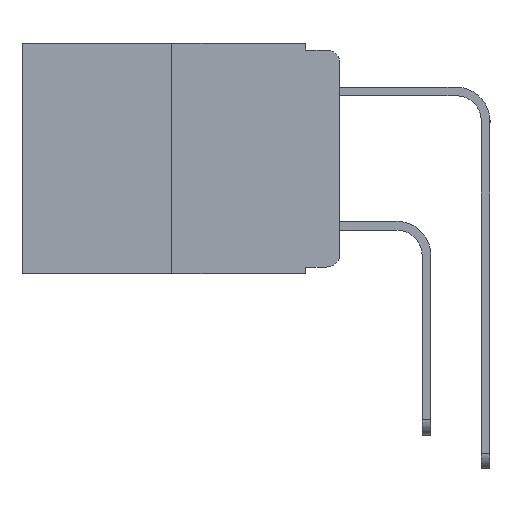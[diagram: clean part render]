
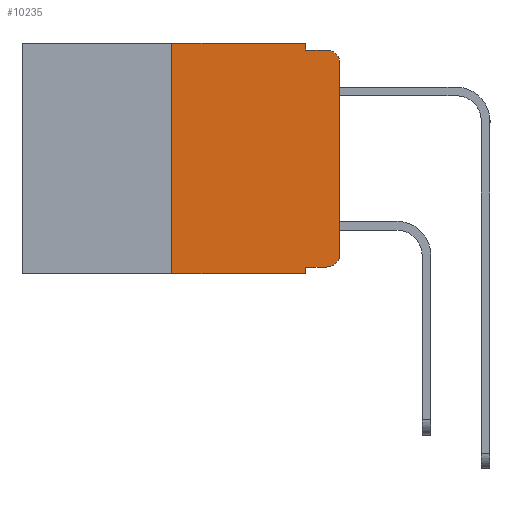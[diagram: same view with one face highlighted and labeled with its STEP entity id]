
A CAD part, left-side view. The second image highlights one B-rep face of the part: STEP entity #10235.
In plain terms, the highlighted planar face has unit normal (-1, 0, 0).
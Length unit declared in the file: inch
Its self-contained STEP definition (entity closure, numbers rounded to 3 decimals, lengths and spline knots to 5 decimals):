
#98 = DIRECTION ( 'NONE',  ( 1., 0., 0. ) ) ;
#112 = LINE ( 'NONE', #6987, #11561 ) ;
#650 = ORIENTED_EDGE ( 'NONE', *, *, #17826, .T. ) ;
#711 = VECTOR ( 'NONE', #14577, 39.37008 ) ;
#1043 = CARTESIAN_POINT ( 'NONE',  ( 0., 0.02, -0.01 ) ) ;
#1067 = EDGE_CURVE ( 'NONE', #17904, #15621, #8961, .T. ) ;
#1271 = CARTESIAN_POINT ( 'NONE',  ( 0., 0.02, -0.313 ) ) ;
#1538 = LINE ( 'NONE', #16977, #8798 ) ;
#1965 = VECTOR ( 'NONE', #10972, 39.37008 ) ;
#2374 = VERTEX_POINT ( 'NONE', #6752 ) ;
#2705 = DIRECTION ( 'NONE',  ( 0., 0., -1. ) ) ;
#2777 = CARTESIAN_POINT ( 'NONE',  ( 0., 0.051, -0.01 ) ) ;
#3746 = LINE ( 'NONE', #13636, #1965 ) ;
#5416 = ORIENTED_EDGE ( 'NONE', *, *, #11792, .F. ) ;
#5908 = VECTOR ( 'NONE', #18033, 39.37008 ) ;
#5997 = ORIENTED_EDGE ( 'NONE', *, *, #6432, .F. ) ;
#6091 = EDGE_CURVE ( 'NONE', #8125, #2374, #15816, .T. ) ;
#6228 = VERTEX_POINT ( 'NONE', #16266 ) ;
#6432 = EDGE_CURVE ( 'NONE', #13119, #15621, #13902, .T. ) ;
#6443 = ORIENTED_EDGE ( 'NONE', *, *, #12571, .F. ) ;
#6477 = VERTEX_POINT ( 'NONE', #11448 ) ;
#6752 = CARTESIAN_POINT ( 'NONE',  ( 0., 0.02, -0.333 ) ) ;
#6987 = CARTESIAN_POINT ( 'NONE',  ( 0., 0.473, 0. ) ) ;
#7459 = ORIENTED_EDGE ( 'NONE', *, *, #9536, .T. ) ;
#7666 = VERTEX_POINT ( 'NONE', #9868 ) ;
#8125 = VERTEX_POINT ( 'NONE', #14861 ) ;
#8144 = VERTEX_POINT ( 'NONE', #10846 ) ;
#8232 = VECTOR ( 'NONE', #13946, 39.37008 ) ;
#8408 = LINE ( 'NONE', #15875, #711 ) ;
#8798 = VECTOR ( 'NONE', #10287, 39.37008 ) ;
#8813 = CARTESIAN_POINT ( 'NONE',  ( 0., 0.473, 0. ) ) ;
#8961 = CIRCLE ( 'NONE', #16165, 0.02 ) ;
#9094 = FACE_OUTER_BOUND ( 'NONE', #17745, .T. ) ;
#9536 = EDGE_CURVE ( 'NONE', #6477, #9588, #11463, .T. ) ;
#9588 = VERTEX_POINT ( 'NONE', #11404 ) ;
#9868 = CARTESIAN_POINT ( 'NONE',  ( 0., 0.25, 0. ) ) ;
#9990 = CARTESIAN_POINT ( 'NONE',  ( 0., 0.473, -0.343 ) ) ;
#10080 = CARTESIAN_POINT ( 'NONE',  ( 0., 0., -0.03 ) ) ;
#10195 = DIRECTION ( 'NONE',  ( 0., 0., -1. ) ) ;
#10235 = ADVANCED_FACE ( 'NONE', ( #9094 ), #15569, .F. ) ;
#10287 = DIRECTION ( 'NONE',  ( 0., 0., -1. ) ) ;
#10846 = CARTESIAN_POINT ( 'NONE',  ( 0., 0.051, 0. ) ) ;
#10972 = DIRECTION ( 'NONE',  ( 0., 0., -1. ) ) ;
#11238 = CARTESIAN_POINT ( 'NONE',  ( 0., 0., 0. ) ) ;
#11264 = DIRECTION ( 'NONE',  ( -1., 0., 0. ) ) ;
#11404 = CARTESIAN_POINT ( 'NONE',  ( 0., 0.051, -0.343 ) ) ;
#11448 = CARTESIAN_POINT ( 'NONE',  ( 0., 0.25, -0.343 ) ) ;
#11463 = LINE ( 'NONE', #9990, #5908 ) ;
#11561 = VECTOR ( 'NONE', #17953, 39.37008 ) ;
#11679 = ORIENTED_EDGE ( 'NONE', *, *, #6091, .T. ) ;
#11792 = EDGE_CURVE ( 'NONE', #8125, #9588, #1538, .T. ) ;
#12025 = DIRECTION ( 'NONE',  ( 0., -1., 0. ) ) ;
#12359 = AXIS2_PLACEMENT_3D ( 'NONE', #8813, #98, #10195 ) ;
#12363 = LINE ( 'NONE', #11238, #8232 ) ;
#12571 = EDGE_CURVE ( 'NONE', #8144, #13119, #3746, .T. ) ;
#12698 = EDGE_CURVE ( 'NONE', #7666, #8144, #112, .T. ) ;
#13119 = VERTEX_POINT ( 'NONE', #16250 ) ;
#13283 = ORIENTED_EDGE ( 'NONE', *, *, #17489, .F. ) ;
#13388 = ORIENTED_EDGE ( 'NONE', *, *, #1067, .T. ) ;
#13636 = CARTESIAN_POINT ( 'NONE',  ( 0., 0.051, 0. ) ) ;
#13901 = EDGE_CURVE ( 'NONE', #6228, #17904, #12363, .T. ) ;
#13902 = LINE ( 'NONE', #2777, #17035 ) ;
#13946 = DIRECTION ( 'NONE',  ( 0., 0., 1. ) ) ;
#14577 = DIRECTION ( 'NONE',  ( 0., 0., 1. ) ) ;
#14861 = CARTESIAN_POINT ( 'NONE',  ( 0., 0.051, -0.333 ) ) ;
#15003 = AXIS2_PLACEMENT_3D ( 'NONE', #1271, #11264, #2705 ) ;
#15148 = ORIENTED_EDGE ( 'NONE', *, *, #12698, .F. ) ;
#15569 = PLANE ( 'NONE',  #12359 ) ;
#15621 = VERTEX_POINT ( 'NONE', #1043 ) ;
#15813 = DIRECTION ( 'NONE',  ( 0., 0., -1. ) ) ;
#15816 = LINE ( 'NONE', #17329, #16220 ) ;
#15819 = DIRECTION ( 'NONE',  ( -1., 0., 0. ) ) ;
#15830 = CARTESIAN_POINT ( 'NONE',  ( 0., 0.02, -0.03 ) ) ;
#15875 = CARTESIAN_POINT ( 'NONE',  ( 0., 0.25, 0. ) ) ;
#16165 = AXIS2_PLACEMENT_3D ( 'NONE', #15830, #15819, #15813 ) ;
#16220 = VECTOR ( 'NONE', #12025, 39.37008 ) ;
#16250 = CARTESIAN_POINT ( 'NONE',  ( 0., 0.051, -0.01 ) ) ;
#16266 = CARTESIAN_POINT ( 'NONE',  ( 0., 0., -0.313 ) ) ;
#16417 = ORIENTED_EDGE ( 'NONE', *, *, #13901, .T. ) ;
#16729 = DIRECTION ( 'NONE',  ( 0., -1., 0. ) ) ;
#16877 = CIRCLE ( 'NONE', #15003, 0.02 ) ;
#16977 = CARTESIAN_POINT ( 'NONE',  ( 0., 0.051, 0. ) ) ;
#17035 = VECTOR ( 'NONE', #16729, 39.37008 ) ;
#17329 = CARTESIAN_POINT ( 'NONE',  ( 0., 0.051, -0.333 ) ) ;
#17489 = EDGE_CURVE ( 'NONE', #6477, #7666, #8408, .T. ) ;
#17745 = EDGE_LOOP ( 'NONE', ( #16417, #13388, #5997, #6443, #15148, #13283, #7459, #5416, #11679, #650 ) ) ;
#17826 = EDGE_CURVE ( 'NONE', #2374, #6228, #16877, .T. ) ;
#17904 = VERTEX_POINT ( 'NONE', #10080 ) ;
#17953 = DIRECTION ( 'NONE',  ( 0., -1., 0. ) ) ;
#18033 = DIRECTION ( 'NONE',  ( 0., -1., 0. ) ) ;
